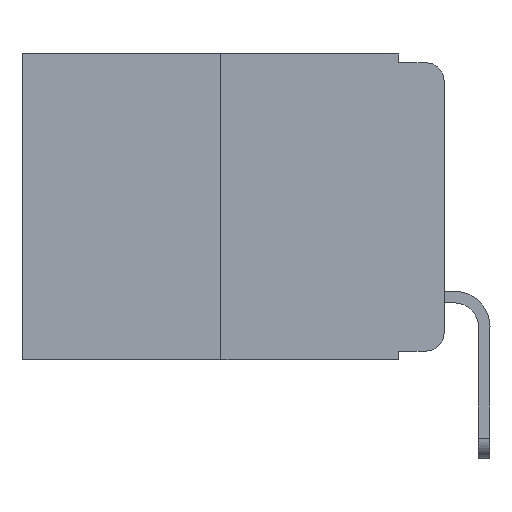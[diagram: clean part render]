
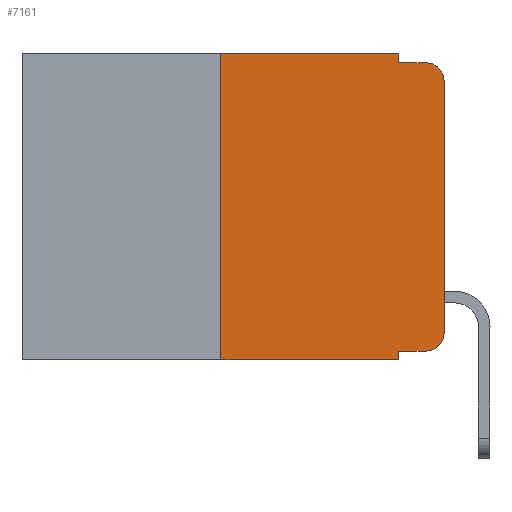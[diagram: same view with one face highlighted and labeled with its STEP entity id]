
A CAD part, left-side view. The second image highlights one B-rep face of the part: STEP entity #7161.
In plain terms, the highlighted planar face has unit normal (-1, 0, 0).
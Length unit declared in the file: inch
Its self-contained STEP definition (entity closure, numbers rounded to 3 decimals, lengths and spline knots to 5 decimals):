
#50 = CARTESIAN_POINT ( 'NONE',  ( 0., 0.02, -0.333 ) ) ;
#107 = DIRECTION ( 'NONE',  ( 0., -1., 0. ) ) ;
#296 = CIRCLE ( 'NONE', #12504, 0.02 ) ;
#541 = CARTESIAN_POINT ( 'NONE',  ( 0., 0.051, -0.01 ) ) ;
#741 = CARTESIAN_POINT ( 'NONE',  ( 0., 0.02, -0.03 ) ) ;
#855 = CARTESIAN_POINT ( 'NONE',  ( 0., 0.051, -0.343 ) ) ;
#1242 = VERTEX_POINT ( 'NONE', #2261 ) ;
#1451 = AXIS2_PLACEMENT_3D ( 'NONE', #8290, #7281, #10412 ) ;
#1601 = VERTEX_POINT ( 'NONE', #9811 ) ;
#1609 = VECTOR ( 'NONE', #7401, 39.37008 ) ;
#1764 = CARTESIAN_POINT ( 'NONE',  ( 0., 0., 0. ) ) ;
#2045 = DIRECTION ( 'NONE',  ( 0., 0., -1. ) ) ;
#2120 = VECTOR ( 'NONE', #10992, 39.37008 ) ;
#2261 = CARTESIAN_POINT ( 'NONE',  ( 0., 0., -0.313 ) ) ;
#2340 = CARTESIAN_POINT ( 'NONE',  ( 0., 0.051, 0. ) ) ;
#2379 = CARTESIAN_POINT ( 'NONE',  ( 0., 0.051, -0.01 ) ) ;
#2573 = ORIENTED_EDGE ( 'NONE', *, *, #7702, .T. ) ;
#2663 = ORIENTED_EDGE ( 'NONE', *, *, #6281, .F. ) ;
#2688 = EDGE_CURVE ( 'NONE', #1242, #9052, #12650, .T. ) ;
#2839 = EDGE_CURVE ( 'NONE', #4870, #9883, #5667, .T. ) ;
#3255 = CIRCLE ( 'NONE', #1451, 0.02 ) ;
#3398 = ORIENTED_EDGE ( 'NONE', *, *, #8909, .T. ) ;
#3465 = DIRECTION ( 'NONE',  ( 0., -1., 0. ) ) ;
#3667 = DIRECTION ( 'NONE',  ( 1., 0., 0. ) ) ;
#4153 = VECTOR ( 'NONE', #2045, 39.37008 ) ;
#4231 = VERTEX_POINT ( 'NONE', #50 ) ;
#4268 = VECTOR ( 'NONE', #9676, 39.37008 ) ;
#4788 = VERTEX_POINT ( 'NONE', #4986 ) ;
#4870 = VERTEX_POINT ( 'NONE', #541 ) ;
#4986 = CARTESIAN_POINT ( 'NONE',  ( 0., 0.051, -0.333 ) ) ;
#5166 = VECTOR ( 'NONE', #107, 39.37008 ) ;
#5667 = LINE ( 'NONE', #2379, #5166 ) ;
#5715 = EDGE_CURVE ( 'NONE', #11315, #13196, #10644, .T. ) ;
#6281 = EDGE_CURVE ( 'NONE', #4788, #13196, #8140, .T. ) ;
#6766 = LINE ( 'NONE', #10675, #1609 ) ;
#6818 = CARTESIAN_POINT ( 'NONE',  ( 0., 0.051, -0.333 ) ) ;
#7132 = VERTEX_POINT ( 'NONE', #2340 ) ;
#7140 = LINE ( 'NONE', #6818, #2120 ) ;
#7161 = ADVANCED_FACE ( 'NONE', ( #11101 ), #11091, .F. ) ;
#7258 = LINE ( 'NONE', #10645, #4268 ) ;
#7281 = DIRECTION ( 'NONE',  ( -1., 0., 0. ) ) ;
#7395 = VECTOR ( 'NONE', #8348, 39.37008 ) ;
#7401 = DIRECTION ( 'NONE',  ( 0., -1., 0. ) ) ;
#7565 = EDGE_LOOP ( 'NONE', ( #9171, #13269, #12639, #9355, #7878, #9619, #13735, #2663, #2573, #3398 ) ) ;
#7702 = EDGE_CURVE ( 'NONE', #4788, #4231, #7140, .T. ) ;
#7878 = ORIENTED_EDGE ( 'NONE', *, *, #12727, .F. ) ;
#8140 = LINE ( 'NONE', #13585, #4153 ) ;
#8183 = DIRECTION ( 'NONE',  ( 0., 0., -1. ) ) ;
#8290 = CARTESIAN_POINT ( 'NONE',  ( 0., 0.02, -0.313 ) ) ;
#8348 = DIRECTION ( 'NONE',  ( 0., 0., 1. ) ) ;
#8909 = EDGE_CURVE ( 'NONE', #4231, #1242, #3255, .T. ) ;
#9052 = VERTEX_POINT ( 'NONE', #11670 ) ;
#9092 = EDGE_CURVE ( 'NONE', #7132, #4870, #7258, .T. ) ;
#9171 = ORIENTED_EDGE ( 'NONE', *, *, #2688, .T. ) ;
#9355 = ORIENTED_EDGE ( 'NONE', *, *, #9092, .F. ) ;
#9619 = ORIENTED_EDGE ( 'NONE', *, *, #10121, .F. ) ;
#9676 = DIRECTION ( 'NONE',  ( 0., 0., -1. ) ) ;
#9709 = LINE ( 'NONE', #10385, #7395 ) ;
#9811 = CARTESIAN_POINT ( 'NONE',  ( 0., 0.25, 0. ) ) ;
#9883 = VERTEX_POINT ( 'NONE', #13100 ) ;
#10018 = DIRECTION ( 'NONE',  ( 0., 0., -1. ) ) ;
#10121 = EDGE_CURVE ( 'NONE', #11315, #1601, #9709, .T. ) ;
#10147 = AXIS2_PLACEMENT_3D ( 'NONE', #11046, #3667, #10018 ) ;
#10252 = DIRECTION ( 'NONE',  ( 0., 0., 1. ) ) ;
#10385 = CARTESIAN_POINT ( 'NONE',  ( 0., 0.25, 0. ) ) ;
#10412 = DIRECTION ( 'NONE',  ( 0., 0., -1. ) ) ;
#10644 = LINE ( 'NONE', #13805, #10982 ) ;
#10645 = CARTESIAN_POINT ( 'NONE',  ( 0., 0.051, 0. ) ) ;
#10675 = CARTESIAN_POINT ( 'NONE',  ( 0., 0.473, 0. ) ) ;
#10816 = VECTOR ( 'NONE', #10252, 39.37008 ) ;
#10982 = VECTOR ( 'NONE', #3465, 39.37008 ) ;
#10992 = DIRECTION ( 'NONE',  ( 0., -1., 0. ) ) ;
#11046 = CARTESIAN_POINT ( 'NONE',  ( 0., 0.473, 0. ) ) ;
#11087 = EDGE_CURVE ( 'NONE', #9052, #9883, #296, .T. ) ;
#11091 = PLANE ( 'NONE',  #10147 ) ;
#11101 = FACE_OUTER_BOUND ( 'NONE', #7565, .T. ) ;
#11315 = VERTEX_POINT ( 'NONE', #12511 ) ;
#11670 = CARTESIAN_POINT ( 'NONE',  ( 0., 0., -0.03 ) ) ;
#12374 = DIRECTION ( 'NONE',  ( -1., 0., 0. ) ) ;
#12504 = AXIS2_PLACEMENT_3D ( 'NONE', #741, #12374, #8183 ) ;
#12511 = CARTESIAN_POINT ( 'NONE',  ( 0., 0.25, -0.343 ) ) ;
#12639 = ORIENTED_EDGE ( 'NONE', *, *, #2839, .F. ) ;
#12650 = LINE ( 'NONE', #1764, #10816 ) ;
#12727 = EDGE_CURVE ( 'NONE', #1601, #7132, #6766, .T. ) ;
#13100 = CARTESIAN_POINT ( 'NONE',  ( 0., 0.02, -0.01 ) ) ;
#13196 = VERTEX_POINT ( 'NONE', #855 ) ;
#13269 = ORIENTED_EDGE ( 'NONE', *, *, #11087, .T. ) ;
#13585 = CARTESIAN_POINT ( 'NONE',  ( 0., 0.051, 0. ) ) ;
#13735 = ORIENTED_EDGE ( 'NONE', *, *, #5715, .T. ) ;
#13805 = CARTESIAN_POINT ( 'NONE',  ( 0., 0.473, -0.343 ) ) ;
